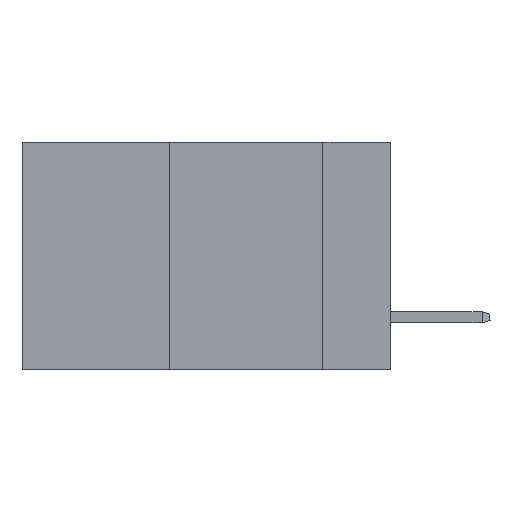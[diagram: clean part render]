
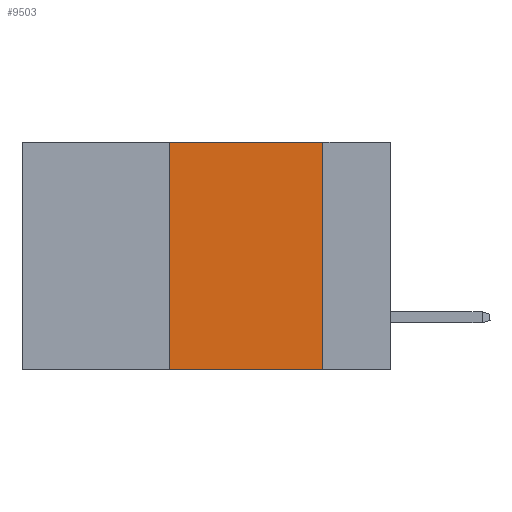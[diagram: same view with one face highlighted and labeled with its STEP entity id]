
A CAD part, left-side view. The second image highlights one B-rep face of the part: STEP entity #9503.
In plain terms, the highlighted planar face has unit normal (-1, 0, 0).
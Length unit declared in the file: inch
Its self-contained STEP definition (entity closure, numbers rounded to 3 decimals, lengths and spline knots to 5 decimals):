
#31 = FACE_OUTER_BOUND ( 'NONE', #22062, .T. ) ;
#162 = VERTEX_POINT ( 'NONE', #20294 ) ;
#310 = ORIENTED_EDGE ( 'NONE', *, *, #7536, .F. ) ;
#895 = VERTEX_POINT ( 'NONE', #4777 ) ;
#1163 = CARTESIAN_POINT ( 'NONE',  ( 0., 0.36, 0. ) ) ;
#2462 = EDGE_CURVE ( 'NONE', #23232, #895, #7283, .T. ) ;
#3070 = CARTESIAN_POINT ( 'NONE',  ( 0., 0.11, 0. ) ) ;
#4777 = CARTESIAN_POINT ( 'NONE',  ( 0., 0.11, 0. ) ) ;
#5000 = DIRECTION ( 'NONE',  ( 0., -1., 0. ) ) ;
#5098 = CARTESIAN_POINT ( 'NONE',  ( 0., 0.6, 0. ) ) ;
#5113 = DIRECTION ( 'NONE',  ( 0., 0., -1. ) ) ;
#5490 = DIRECTION ( 'NONE',  ( 0., 0., -1. ) ) ;
#5657 = DIRECTION ( 'NONE',  ( 1., 0., 0. ) ) ;
#7283 = LINE ( 'NONE', #5098, #10110 ) ;
#7536 = EDGE_CURVE ( 'NONE', #162, #23232, #15362, .T. ) ;
#8367 = LINE ( 'NONE', #3070, #20152 ) ;
#9503 = ADVANCED_FACE ( 'NONE', ( #31 ), #21626, .F. ) ;
#10110 = VECTOR ( 'NONE', #5000, 39.37008 ) ;
#10169 = VERTEX_POINT ( 'NONE', #19030 ) ;
#10697 = VECTOR ( 'NONE', #14950, 39.37008 ) ;
#11550 = VECTOR ( 'NONE', #23403, 39.37008 ) ;
#12827 = CARTESIAN_POINT ( 'NONE',  ( 0., 0.36, 0. ) ) ;
#14950 = DIRECTION ( 'NONE',  ( 0., -1., 0. ) ) ;
#15362 = LINE ( 'NONE', #1163, #11550 ) ;
#17980 = EDGE_CURVE ( 'NONE', #895, #10169, #8367, .T. ) ;
#19030 = CARTESIAN_POINT ( 'NONE',  ( 0., 0.11, -0.37 ) ) ;
#20152 = VECTOR ( 'NONE', #5113, 39.37008 ) ;
#20294 = CARTESIAN_POINT ( 'NONE',  ( 0., 0.36, -0.37 ) ) ;
#20824 = ORIENTED_EDGE ( 'NONE', *, *, #17980, .F. ) ;
#21612 = AXIS2_PLACEMENT_3D ( 'NONE', #23970, #5657, #5490 ) ;
#21626 = PLANE ( 'NONE',  #21612 ) ;
#22062 = EDGE_LOOP ( 'NONE', ( #20824, #23868, #310, #24458 ) ) ;
#22630 = EDGE_CURVE ( 'NONE', #162, #10169, #25860, .T. ) ;
#23232 = VERTEX_POINT ( 'NONE', #12827 ) ;
#23403 = DIRECTION ( 'NONE',  ( 0., 0., 1. ) ) ;
#23868 = ORIENTED_EDGE ( 'NONE', *, *, #2462, .F. ) ;
#23970 = CARTESIAN_POINT ( 'NONE',  ( 0., 0.6, 0. ) ) ;
#24458 = ORIENTED_EDGE ( 'NONE', *, *, #22630, .T. ) ;
#24889 = CARTESIAN_POINT ( 'NONE',  ( 0., 0.6, -0.37 ) ) ;
#25860 = LINE ( 'NONE', #24889, #10697 ) ;
